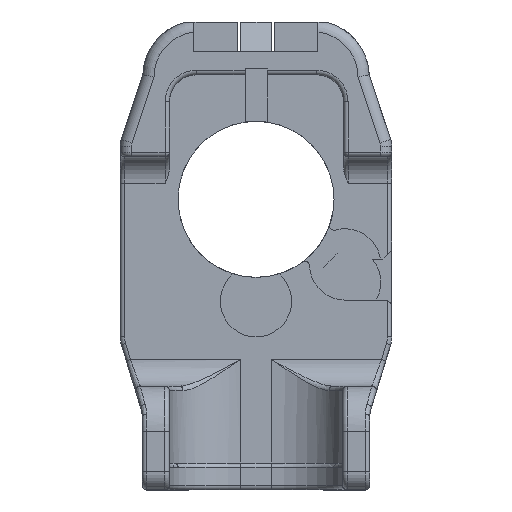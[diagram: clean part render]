
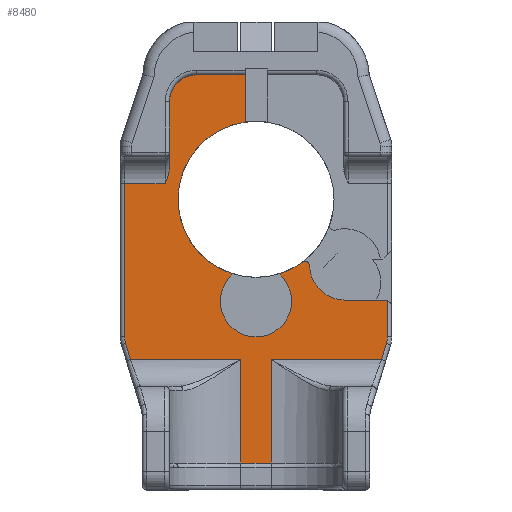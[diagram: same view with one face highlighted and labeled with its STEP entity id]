
A CAD part, front view. The second image highlights one B-rep face of the part: STEP entity #8480.
In plain terms, the highlighted planar face has unit normal (0, -1, 0).
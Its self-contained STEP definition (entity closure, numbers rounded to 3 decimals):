
#165=PLANE('',#9090);
#463=FACE_OUTER_BOUND('',#973,.T.);
#973=EDGE_LOOP('',(#6045,#6046,#6047,#6048,#6049,#6050,#6051,#6052,#6053,
#6054,#6055,#6056,#6057,#6058,#6059,#6060,#6061,#6062,#6063,#6064,#6065,
#6066,#6067));
#1463=B_SPLINE_CURVE_WITH_KNOTS('',3,(#13048,#13049,#13050,#13051),
 .UNSPECIFIED.,.F.,.F.,(4,4),(0.382,0.56),
 .UNSPECIFIED.);
#1700=LINE('',#12674,#2509);
#1705=LINE('',#12685,#2514);
#1753=LINE('',#12903,#2562);
#1754=LINE('',#12908,#2563);
#1779=LINE('',#13037,#2588);
#1780=LINE('',#13040,#2589);
#1781=LINE('',#13042,#2590);
#1782=LINE('',#13046,#2591);
#1783=LINE('',#13053,#2592);
#1784=LINE('',#13055,#2593);
#1785=LINE('',#13059,#2594);
#1786=LINE('',#13060,#2595);
#1787=LINE('',#13062,#2596);
#1788=LINE('',#13064,#2597);
#2509=VECTOR('',#9895,10.);
#2514=VECTOR('',#9904,10.);
#2562=VECTOR('',#10082,10.);
#2563=VECTOR('',#10087,10.);
#2588=VECTOR('',#10162,10.);
#2589=VECTOR('',#10165,10.);
#2590=VECTOR('',#10166,10.);
#2591=VECTOR('',#10169,10.);
#2592=VECTOR('',#10170,10.);
#2593=VECTOR('',#10171,10.);
#2594=VECTOR('',#10174,10.);
#2595=VECTOR('',#10175,10.);
#2596=VECTOR('',#10176,10.);
#2597=VECTOR('',#10177,10.);
#3270=CIRCLE('',#8966,8.75);
#3272=CIRCLE('',#8968,8.75);
#3291=CIRCLE('',#8991,0.5);
#3295=CIRCLE('',#9001,4.);
#3299=CIRCLE('',#9009,4.);
#3343=CIRCLE('',#9091,5.08);
#3344=CIRCLE('',#9092,2.5);
#3345=CIRCLE('',#9093,2.5);
#3585=VERTEX_POINT('',#12297);
#3586=VERTEX_POINT('',#12299);
#3589=VERTEX_POINT('',#12305);
#3590=VERTEX_POINT('',#12307);
#3656=VERTEX_POINT('',#12661);
#3658=VERTEX_POINT('',#12667);
#3660=VERTEX_POINT('',#12673);
#3664=VERTEX_POINT('',#12683);
#3731=VERTEX_POINT('',#12890);
#3733=VERTEX_POINT('',#12894);
#3734=VERTEX_POINT('',#12905);
#3735=VERTEX_POINT('',#12907);
#3763=VERTEX_POINT('',#13039);
#3764=VERTEX_POINT('',#13041);
#3765=VERTEX_POINT('',#13043);
#3766=VERTEX_POINT('',#13045);
#3767=VERTEX_POINT('',#13047);
#3768=VERTEX_POINT('',#13052);
#3769=VERTEX_POINT('',#13054);
#3770=VERTEX_POINT('',#13056);
#3771=VERTEX_POINT('',#13058);
#3772=VERTEX_POINT('',#13061);
#3773=VERTEX_POINT('',#13063);
#4395=EDGE_CURVE('',#3586,#3585,#3270,.T.);
#4399=EDGE_CURVE('',#3590,#3589,#3272,.T.);
#4469=EDGE_CURVE('',#3590,#3656,#3291,.T.);
#4475=EDGE_CURVE('',#3658,#3660,#1700,.T.);
#4481=EDGE_CURVE('',#3664,#3658,#1705,.T.);
#4485=EDGE_CURVE('',#3664,#3656,#3295,.T.);
#4499=EDGE_CURVE('',#3589,#3586,#3299,.T.);
#4575=EDGE_CURVE('',#3733,#3731,#1753,.T.);
#4577=EDGE_CURVE('',#3734,#3735,#1754,.T.);
#4618=EDGE_CURVE('',#3734,#3731,#1779,.T.);
#4619=EDGE_CURVE('',#3585,#3763,#1780,.T.);
#4620=EDGE_CURVE('',#3764,#3763,#1781,.T.);
#4621=EDGE_CURVE('',#3764,#3765,#3343,.T.);
#4622=EDGE_CURVE('',#3765,#3766,#1782,.T.);
#4623=EDGE_CURVE('',#3767,#3766,#1463,.F.);
#4624=EDGE_CURVE('',#3768,#3767,#1783,.T.);
#4625=EDGE_CURVE('',#3769,#3768,#1784,.T.);
#4626=EDGE_CURVE('',#3770,#3769,#3344,.T.);
#4627=EDGE_CURVE('',#3771,#3770,#1785,.T.);
#4628=EDGE_CURVE('',#3771,#3735,#1786,.T.);
#4629=EDGE_CURVE('',#3733,#3772,#1787,.T.);
#4630=EDGE_CURVE('',#3773,#3772,#1788,.T.);
#4631=EDGE_CURVE('',#3660,#3773,#3345,.T.);
#6045=ORIENTED_EDGE('',*,*,#4469,.F.);
#6046=ORIENTED_EDGE('',*,*,#4399,.T.);
#6047=ORIENTED_EDGE('',*,*,#4499,.T.);
#6048=ORIENTED_EDGE('',*,*,#4395,.T.);
#6049=ORIENTED_EDGE('',*,*,#4619,.T.);
#6050=ORIENTED_EDGE('',*,*,#4620,.F.);
#6051=ORIENTED_EDGE('',*,*,#4621,.T.);
#6052=ORIENTED_EDGE('',*,*,#4622,.T.);
#6053=ORIENTED_EDGE('',*,*,#4623,.F.);
#6054=ORIENTED_EDGE('',*,*,#4624,.F.);
#6055=ORIENTED_EDGE('',*,*,#4625,.F.);
#6056=ORIENTED_EDGE('',*,*,#4626,.F.);
#6057=ORIENTED_EDGE('',*,*,#4627,.F.);
#6058=ORIENTED_EDGE('',*,*,#4628,.T.);
#6059=ORIENTED_EDGE('',*,*,#4577,.F.);
#6060=ORIENTED_EDGE('',*,*,#4618,.T.);
#6061=ORIENTED_EDGE('',*,*,#4575,.F.);
#6062=ORIENTED_EDGE('',*,*,#4629,.T.);
#6063=ORIENTED_EDGE('',*,*,#4630,.F.);
#6064=ORIENTED_EDGE('',*,*,#4631,.F.);
#6065=ORIENTED_EDGE('',*,*,#4475,.F.);
#6066=ORIENTED_EDGE('',*,*,#4481,.F.);
#6067=ORIENTED_EDGE('',*,*,#4485,.T.);
#8480=ADVANCED_FACE('',(#463),#165,.T.);
#8966=AXIS2_PLACEMENT_3D('',#12300,#9798,#9799);
#8968=AXIS2_PLACEMENT_3D('',#12308,#9804,#9805);
#8991=AXIS2_PLACEMENT_3D('',#12662,#9882,#9883);
#9001=AXIS2_PLACEMENT_3D('',#12693,#9913,#9914);
#9009=AXIS2_PLACEMENT_3D('',#12723,#9938,#9939);
#9090=AXIS2_PLACEMENT_3D('',#13038,#10163,#10164);
#9091=AXIS2_PLACEMENT_3D('',#13044,#10167,#10168);
#9092=AXIS2_PLACEMENT_3D('',#13057,#10172,#10173);
#9093=AXIS2_PLACEMENT_3D('',#13065,#10178,#10179);
#9798=DIRECTION('center_axis',(0.,1.,0.));
#9799=DIRECTION('ref_axis',(-1.,0.,0.));
#9804=DIRECTION('center_axis',(0.,1.,0.));
#9805=DIRECTION('ref_axis',(-1.,0.,0.));
#9882=DIRECTION('center_axis',(0.,1.,0.));
#9883=DIRECTION('ref_axis',(0.437,0.,0.9));
#9895=DIRECTION('',(0.,0.,-1.));
#9904=DIRECTION('',(1.,0.,0.));
#9913=DIRECTION('center_axis',(0.,1.,0.));
#9914=DIRECTION('ref_axis',(-0.751,0.,0.66));
#9938=DIRECTION('center_axis',(0.,1.,0.));
#9939=DIRECTION('ref_axis',(1.,0.,0.));
#10082=DIRECTION('',(0.,0.,-1.));
#10087=DIRECTION('',(0.,0.,1.));
#10162=DIRECTION('',(1.,0.,0.));
#10163=DIRECTION('center_axis',(0.,-1.,0.));
#10164=DIRECTION('ref_axis',(0.,0.,-1.));
#10165=DIRECTION('',(0.,0.,1.));
#10166=DIRECTION('',(1.,0.,0.));
#10167=DIRECTION('center_axis',(0.,-1.,0.));
#10168=DIRECTION('ref_axis',(-0.707,0.,0.707));
#10169=DIRECTION('',(0.,0.,-1.));
#10170=DIRECTION('',(1.,0.,0.));
#10171=DIRECTION('',(0.,0.,1.));
#10172=DIRECTION('center_axis',(0.,1.,0.));
#10173=DIRECTION('ref_axis',(-0.989,0.,-0.149));
#10174=DIRECTION('',(-0.294,0.,0.956));
#10175=DIRECTION('',(1.,0.,0.));
#10176=DIRECTION('',(1.,0.,0.));
#10177=DIRECTION('',(-0.294,0.,-0.956));
#10178=DIRECTION('center_axis',(0.,1.,0.));
#10179=DIRECTION('ref_axis',(0.989,0.,-0.149));
#12297=CARTESIAN_POINT('',(-1.212,65.024,-4.904));
#12299=CARTESIAN_POINT('',(-2.569,65.024,-21.934));
#12300=CARTESIAN_POINT('Origin',(0.,65.024,-13.57));
#12305=CARTESIAN_POINT('',(2.569,65.024,-21.934));
#12307=CARTESIAN_POINT('',(5.205,65.024,-20.604));
#12308=CARTESIAN_POINT('Origin',(0.,65.024,-13.57));
#12661=CARTESIAN_POINT('',(6.002,65.024,-20.991));
#12662=CARTESIAN_POINT('Origin',(5.502,65.024,-21.006));
#12667=CARTESIAN_POINT('',(14.74,65.024,-24.871));
#12673=CARTESIAN_POINT('',(14.74,65.024,-28.994));
#12674=CARTESIAN_POINT('',(14.74,65.024,-15.945));
#12683=CARTESIAN_POINT('',(9.906,65.024,-24.871));
#12685=CARTESIAN_POINT('',(9.953,65.024,-24.871));
#12693=CARTESIAN_POINT('Origin',(10.,65.024,-20.872));
#12723=CARTESIAN_POINT('Origin',(0.,65.024,-25.));
#12890=CARTESIAN_POINT('',(1.723,65.024,-43.145));
#12894=CARTESIAN_POINT('',(1.723,65.024,-31.525));
#12903=CARTESIAN_POINT('',(1.723,65.024,-26.066));
#12905=CARTESIAN_POINT('',(-1.723,65.024,-43.145));
#12907=CARTESIAN_POINT('',(-1.723,65.024,-31.525));
#12908=CARTESIAN_POINT('',(-1.723,65.024,-33.763));
#13037=CARTESIAN_POINT('',(-6.35,65.024,-43.145));
#13038=CARTESIAN_POINT('Origin',(-12.7,65.024,-17.382));
#13039=CARTESIAN_POINT('',(-1.212,65.024,0.394));
#13040=CARTESIAN_POINT('',(-1.212,65.024,-11.281));
#13041=CARTESIAN_POINT('',(-7.62,65.024,0.394));
#13042=CARTESIAN_POINT('',(-12.701,65.024,0.394));
#13043=CARTESIAN_POINT('',(-9.692,65.024,-0.048));
#13044=CARTESIAN_POINT('Origin',(-7.62,65.024,-4.686));
#13045=CARTESIAN_POINT('',(-9.692,65.024,-10.002));
#13046=CARTESIAN_POINT('',(-9.692,65.024,-13.093));
#13047=CARTESIAN_POINT('',(-10.192,65.024,-11.805));
#13048=CARTESIAN_POINT('Ctrl Pts',(-9.692,65.024,-10.002));
#13049=CARTESIAN_POINT('Ctrl Pts',(-9.692,65.024,-10.597));
#13050=CARTESIAN_POINT('Ctrl Pts',(-9.968,65.024,-11.255));
#13051=CARTESIAN_POINT('Ctrl Pts',(-10.192,65.024,-11.805));
#13052=CARTESIAN_POINT('',(-14.74,65.024,-11.805));
#13053=CARTESIAN_POINT('',(-13.97,65.024,-11.805));
#13054=CARTESIAN_POINT('',(-14.74,65.024,-28.994));
#13055=CARTESIAN_POINT('',(-14.74,65.024,-15.95));
#13056=CARTESIAN_POINT('',(-14.629,65.024,-29.729));
#13057=CARTESIAN_POINT('Origin',(-12.24,65.024,-28.994));
#13058=CARTESIAN_POINT('',(-14.077,65.024,-31.525));
#13059=CARTESIAN_POINT('',(-15.078,65.024,-28.272));
#13060=CARTESIAN_POINT('',(-10.795,65.024,-31.525));
#13061=CARTESIAN_POINT('',(14.077,65.024,-31.525));
#13062=CARTESIAN_POINT('',(1.27,65.024,-31.525));
#13063=CARTESIAN_POINT('',(14.629,65.024,-29.729));
#13064=CARTESIAN_POINT('',(16.519,65.024,-23.587));
#13065=CARTESIAN_POINT('Origin',(12.24,65.024,-28.994));
